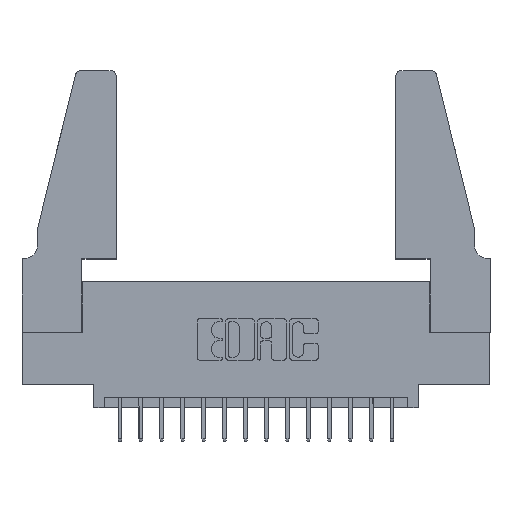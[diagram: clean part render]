
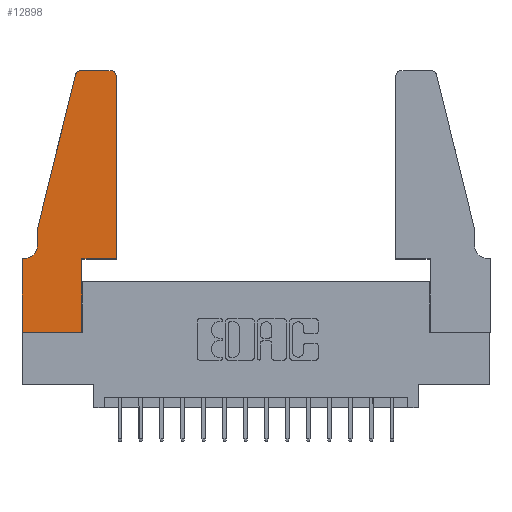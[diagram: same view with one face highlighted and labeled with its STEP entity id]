
A CAD part, top view. The second image highlights one B-rep face of the part: STEP entity #12898.
In plain terms, the highlighted planar face has unit normal (0, 0, 1).
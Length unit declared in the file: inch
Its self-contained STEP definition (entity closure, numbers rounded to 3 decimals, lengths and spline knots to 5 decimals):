
#190 = ORIENTED_EDGE ( 'NONE', *, *, #15772, .T. ) ;
#333 = EDGE_CURVE ( 'NONE', #2227, #11933, #15166, .T. ) ;
#548 = CARTESIAN_POINT ( 'NONE',  ( 0., 0.35, 0.37 ) ) ;
#631 = LINE ( 'NONE', #2831, #13395 ) ;
#685 = EDGE_LOOP ( 'NONE', ( #1965, #16302, #190, #10941, #16375, #12355, #14935, #2788, #3524, #8752, #5659, #9944 ) ) ;
#838 = EDGE_CURVE ( 'NONE', #5164, #7798, #7410, .T. ) ;
#895 = VECTOR ( 'NONE', #3459, 39.37008 ) ;
#918 = CARTESIAN_POINT ( 'NONE',  ( 0.0055, 0.35, 0.37 ) ) ;
#1568 = CARTESIAN_POINT ( 'NONE',  ( 0.0755, 0.5, 0.37 ) ) ;
#1685 = FACE_OUTER_BOUND ( 'NONE', #685, .T. ) ;
#1944 = CARTESIAN_POINT ( 'NONE',  ( 0.0755, 0.35, 0.37 ) ) ;
#1965 = ORIENTED_EDGE ( 'NONE', *, *, #7833, .T. ) ;
#2095 = VERTEX_POINT ( 'NONE', #10435 ) ;
#2227 = VERTEX_POINT ( 'NONE', #13920 ) ;
#2788 = ORIENTED_EDGE ( 'NONE', *, *, #15261, .T. ) ;
#2831 = CARTESIAN_POINT ( 'NONE',  ( 0.4505, 0.35, 0.37 ) ) ;
#3259 = DIRECTION ( 'NONE',  ( 0., 0., -1. ) ) ;
#3308 = VERTEX_POINT ( 'NONE', #14876 ) ;
#3326 = VECTOR ( 'NONE', #16955, 39.37008 ) ;
#3459 = DIRECTION ( 'NONE',  ( -1., 0., 0. ) ) ;
#3503 = AXIS2_PLACEMENT_3D ( 'NONE', #15985, #5471, #14561 ) ;
#3524 = ORIENTED_EDGE ( 'NONE', *, *, #838, .T. ) ;
#3539 = CARTESIAN_POINT ( 'NONE',  ( 0.2865, 0.35, 0.37 ) ) ;
#3554 = DIRECTION ( 'NONE',  ( 1., 0., 0. ) ) ;
#4178 = CARTESIAN_POINT ( 'NONE',  ( 0., 0.35, 0.37 ) ) ;
#4826 = CARTESIAN_POINT ( 'NONE',  ( 0.2605, 1.25, 0.37 ) ) ;
#5091 = CARTESIAN_POINT ( 'NONE',  ( 0.2865, 0., 0.37 ) ) ;
#5164 = VERTEX_POINT ( 'NONE', #5091 ) ;
#5244 = AXIS2_PLACEMENT_3D ( 'NONE', #4178, #16279, #9584 ) ;
#5471 = DIRECTION ( 'NONE',  ( 0., 0., 1. ) ) ;
#5493 = EDGE_CURVE ( 'NONE', #5657, #15530, #15959, .T. ) ;
#5657 = VERTEX_POINT ( 'NONE', #918 ) ;
#5659 = ORIENTED_EDGE ( 'NONE', *, *, #7760, .T. ) ;
#6271 = DIRECTION ( 'NONE',  ( -1., 0., 0. ) ) ;
#6589 = CARTESIAN_POINT ( 'NONE',  ( 0.4205, 1.22, 0.37 ) ) ;
#6757 = VERTEX_POINT ( 'NONE', #16777 ) ;
#6981 = VECTOR ( 'NONE', #10322, 39.37008 ) ;
#7021 = CARTESIAN_POINT ( 'NONE',  ( 0., 0., 0.37 ) ) ;
#7410 = LINE ( 'NONE', #12454, #6981 ) ;
#7452 = CARTESIAN_POINT ( 'NONE',  ( 0.4505, 0.35, 0.37 ) ) ;
#7489 = LINE ( 'NONE', #7452, #13885 ) ;
#7494 = CARTESIAN_POINT ( 'NONE',  ( 0.25487, 1.22718, 0.37 ) ) ;
#7760 = EDGE_CURVE ( 'NONE', #2095, #9638, #631, .T. ) ;
#7798 = VERTEX_POINT ( 'NONE', #3539 ) ;
#7833 = EDGE_CURVE ( 'NONE', #6757, #2227, #14019, .T. ) ;
#8129 = CARTESIAN_POINT ( 'NONE',  ( 0., 0., 0.37 ) ) ;
#8678 = CARTESIAN_POINT ( 'NONE',  ( 0.0755, 0.5, 0.37 ) ) ;
#8752 = ORIENTED_EDGE ( 'NONE', *, *, #11435, .T. ) ;
#8808 = CARTESIAN_POINT ( 'NONE',  ( 0., 0., 0.37 ) ) ;
#8972 = VERTEX_POINT ( 'NONE', #8678 ) ;
#9378 = EDGE_CURVE ( 'NONE', #8972, #3308, #9824, .T. ) ;
#9584 = DIRECTION ( 'NONE',  ( 1., 0., 0. ) ) ;
#9638 = VERTEX_POINT ( 'NONE', #15553 ) ;
#9709 = VECTOR ( 'NONE', #10854, 39.37008 ) ;
#9824 = LINE ( 'NONE', #1568, #12126 ) ;
#9861 = DIRECTION ( 'NONE',  ( -1., 0., 0. ) ) ;
#9944 = ORIENTED_EDGE ( 'NONE', *, *, #16524, .T. ) ;
#10322 = DIRECTION ( 'NONE',  ( 0., 1., 0. ) ) ;
#10367 = CARTESIAN_POINT ( 'NONE',  ( 0.0755, 0.5, 0.37 ) ) ;
#10435 = CARTESIAN_POINT ( 'NONE',  ( 0.4505, 0.35, 0.37 ) ) ;
#10543 = LINE ( 'NONE', #8129, #9709 ) ;
#10641 = PLANE ( 'NONE',  #5244 ) ;
#10854 = DIRECTION ( 'NONE',  ( 1., 0., 0. ) ) ;
#10916 = DIRECTION ( 'NONE',  ( 0., -1., 0. ) ) ;
#10917 = VECTOR ( 'NONE', #6271, 39.37008 ) ;
#10941 = ORIENTED_EDGE ( 'NONE', *, *, #9378, .T. ) ;
#11140 = CARTESIAN_POINT ( 'NONE',  ( 0.0055, 0.42, 0.37 ) ) ;
#11429 = DIRECTION ( 'NONE',  ( 0., 1., 0. ) ) ;
#11435 = EDGE_CURVE ( 'NONE', #7798, #2095, #7489, .T. ) ;
#11922 = AXIS2_PLACEMENT_3D ( 'NONE', #6589, #14634, #15814 ) ;
#11933 = VERTEX_POINT ( 'NONE', #7494 ) ;
#12078 = CIRCLE ( 'NONE', #13292, 0.07 ) ;
#12126 = VECTOR ( 'NONE', #10916, 39.37008 ) ;
#12195 = LINE ( 'NONE', #10367, #3326 ) ;
#12355 = ORIENTED_EDGE ( 'NONE', *, *, #5493, .T. ) ;
#12454 = CARTESIAN_POINT ( 'NONE',  ( 0.2865, 0.35, 0.37 ) ) ;
#12637 = VERTEX_POINT ( 'NONE', #8808 ) ;
#12898 = ADVANCED_FACE ( 'NONE', ( #1685 ), #10641, .T. ) ;
#13292 = AXIS2_PLACEMENT_3D ( 'NONE', #11140, #3259, #9861 ) ;
#13395 = VECTOR ( 'NONE', #11429, 39.37008 ) ;
#13744 = EDGE_CURVE ( 'NONE', #3308, #5657, #12078, .T. ) ;
#13885 = VECTOR ( 'NONE', #3554, 39.37008 ) ;
#13920 = CARTESIAN_POINT ( 'NONE',  ( 0.284, 1.25, 0.37 ) ) ;
#14019 = LINE ( 'NONE', #4826, #10917 ) ;
#14561 = DIRECTION ( 'NONE',  ( 1., 0., 0. ) ) ;
#14634 = DIRECTION ( 'NONE',  ( 0., 0., 1. ) ) ;
#14676 = VECTOR ( 'NONE', #15088, 39.37008 ) ;
#14876 = CARTESIAN_POINT ( 'NONE',  ( 0.0755, 0.42, 0.37 ) ) ;
#14935 = ORIENTED_EDGE ( 'NONE', *, *, #15388, .T. ) ;
#15088 = DIRECTION ( 'NONE',  ( 0., -1., 0. ) ) ;
#15166 = CIRCLE ( 'NONE', #3503, 0.03 ) ;
#15261 = EDGE_CURVE ( 'NONE', #12637, #5164, #10543, .T. ) ;
#15388 = EDGE_CURVE ( 'NONE', #15530, #12637, #16368, .T. ) ;
#15530 = VERTEX_POINT ( 'NONE', #548 ) ;
#15553 = CARTESIAN_POINT ( 'NONE',  ( 0.4505, 1.22, 0.37 ) ) ;
#15772 = EDGE_CURVE ( 'NONE', #11933, #8972, #12195, .T. ) ;
#15814 = DIRECTION ( 'NONE',  ( 1., 0., 0. ) ) ;
#15959 = LINE ( 'NONE', #1944, #895 ) ;
#15985 = CARTESIAN_POINT ( 'NONE',  ( 0.284, 1.22, 0.37 ) ) ;
#16279 = DIRECTION ( 'NONE',  ( 0., 0., 1. ) ) ;
#16302 = ORIENTED_EDGE ( 'NONE', *, *, #333, .T. ) ;
#16368 = LINE ( 'NONE', #7021, #14676 ) ;
#16375 = ORIENTED_EDGE ( 'NONE', *, *, #13744, .T. ) ;
#16524 = EDGE_CURVE ( 'NONE', #9638, #6757, #16529, .T. ) ;
#16529 = CIRCLE ( 'NONE', #11922, 0.03 ) ;
#16777 = CARTESIAN_POINT ( 'NONE',  ( 0.4205, 1.25, 0.37 ) ) ;
#16955 = DIRECTION ( 'NONE',  ( -0.239, -0.971, 0. ) ) ;
